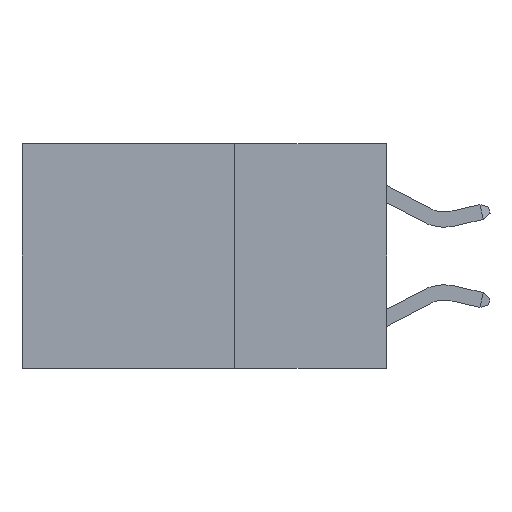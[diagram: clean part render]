
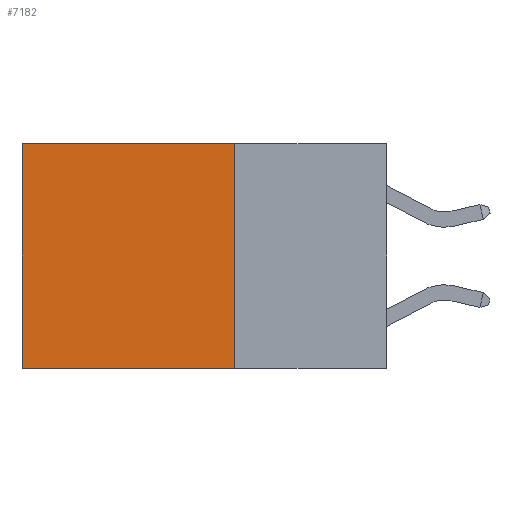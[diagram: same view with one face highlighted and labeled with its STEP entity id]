
A CAD part, left-side view. The second image highlights one B-rep face of the part: STEP entity #7182.
In plain terms, the highlighted planar face has unit normal (-1, 0, 0).
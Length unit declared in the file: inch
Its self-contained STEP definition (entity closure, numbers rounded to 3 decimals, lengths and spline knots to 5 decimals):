
#226 = ORIENTED_EDGE ( 'NONE', *, *, #10253, .T. ) ;
#250 = ORIENTED_EDGE ( 'NONE', *, *, #434, .F. ) ;
#274 = ORIENTED_EDGE ( 'NONE', *, *, #9284, .F. ) ;
#310 = LINE ( 'NONE', #9741, #9598 ) ;
#377 = ORIENTED_EDGE ( 'NONE', *, *, #5937, .T. ) ;
#434 = EDGE_CURVE ( 'NONE', #3767, #5308, #6826, .T. ) ;
#1292 = DIRECTION ( 'NONE',  ( 1., 0., 0. ) ) ;
#1767 = VERTEX_POINT ( 'NONE', #9804 ) ;
#2649 = EDGE_LOOP ( 'NONE', ( #226, #250, #274, #377 ) ) ;
#3286 = CARTESIAN_POINT ( 'NONE',  ( 0.2625, 0.6, 0. ) ) ;
#3748 = DIRECTION ( 'NONE',  ( 0., 1., 0. ) ) ;
#3767 = VERTEX_POINT ( 'NONE', #5958 ) ;
#4356 = LINE ( 'NONE', #3286, #10529 ) ;
#4407 = AXIS2_PLACEMENT_3D ( 'NONE', #8312, #1292, #7572 ) ;
#4585 = LINE ( 'NONE', #9949, #6603 ) ;
#5308 = VERTEX_POINT ( 'NONE', #5727 ) ;
#5727 = CARTESIAN_POINT ( 'NONE',  ( 0.2625, 0.6, -0.37 ) ) ;
#5937 = EDGE_CURVE ( 'NONE', #1767, #6544, #4585, .T. ) ;
#5958 = CARTESIAN_POINT ( 'NONE',  ( 0.2625, 0.25, -0.37 ) ) ;
#6097 = FACE_OUTER_BOUND ( 'NONE', #2649, .T. ) ;
#6163 = CARTESIAN_POINT ( 'NONE',  ( 0.2625, 0.6, 0. ) ) ;
#6544 = VERTEX_POINT ( 'NONE', #6163 ) ;
#6574 = VECTOR ( 'NONE', #3748, 39.37008 ) ;
#6603 = VECTOR ( 'NONE', #9982, 39.37008 ) ;
#6794 = PLANE ( 'NONE',  #4407 ) ;
#6826 = LINE ( 'NONE', #10501, #6574 ) ;
#7182 = ADVANCED_FACE ( 'NONE', ( #6097 ), #6794, .F. ) ;
#7572 = DIRECTION ( 'NONE',  ( 0., 0., -1. ) ) ;
#8168 = DIRECTION ( 'NONE',  ( 0., 0., -1. ) ) ;
#8312 = CARTESIAN_POINT ( 'NONE',  ( 0.2625, 0.25, 0. ) ) ;
#9284 = EDGE_CURVE ( 'NONE', #1767, #3767, #310, .T. ) ;
#9598 = VECTOR ( 'NONE', #8168, 39.37008 ) ;
#9741 = CARTESIAN_POINT ( 'NONE',  ( 0.2625, 0.25, 0. ) ) ;
#9804 = CARTESIAN_POINT ( 'NONE',  ( 0.2625, 0.25, 0. ) ) ;
#9937 = DIRECTION ( 'NONE',  ( 0., 0., -1. ) ) ;
#9949 = CARTESIAN_POINT ( 'NONE',  ( 0.2625, 0.25, 0. ) ) ;
#9982 = DIRECTION ( 'NONE',  ( 0., 1., 0. ) ) ;
#10253 = EDGE_CURVE ( 'NONE', #6544, #5308, #4356, .T. ) ;
#10501 = CARTESIAN_POINT ( 'NONE',  ( 0.2625, 0.25, -0.37 ) ) ;
#10529 = VECTOR ( 'NONE', #9937, 39.37008 ) ;
